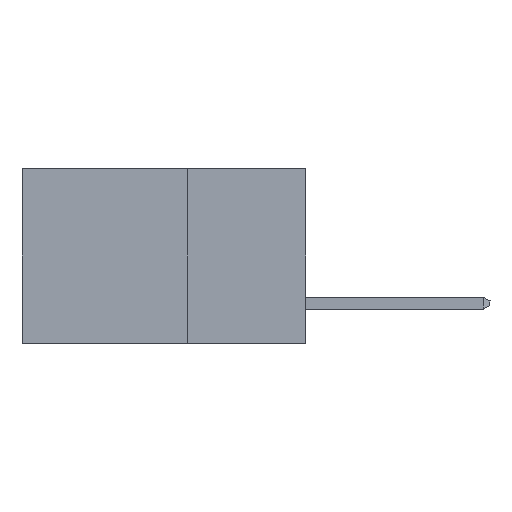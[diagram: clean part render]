
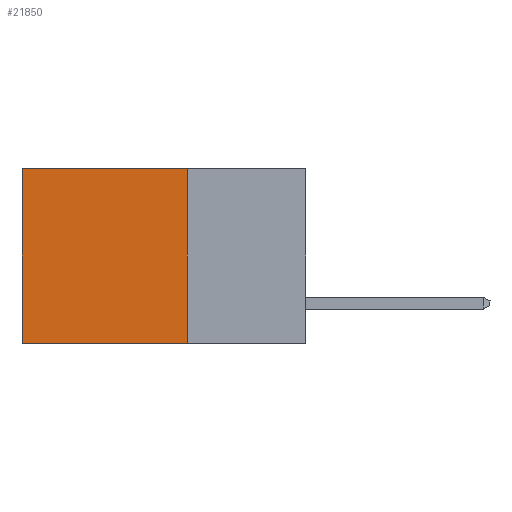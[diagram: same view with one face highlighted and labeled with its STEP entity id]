
A CAD part, left-side view. The second image highlights one B-rep face of the part: STEP entity #21850.
In plain terms, the highlighted planar face has unit normal (-1, 0, 0).
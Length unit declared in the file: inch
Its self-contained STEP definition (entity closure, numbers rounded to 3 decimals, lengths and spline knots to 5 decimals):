
#403 = VERTEX_POINT ( 'NONE', #14702 ) ;
#495 = AXIS2_PLACEMENT_3D ( 'NONE', #4971, #12656, #16238 ) ;
#599 = FACE_OUTER_BOUND ( 'NONE', #5117, .T. ) ;
#920 = DIRECTION ( 'NONE',  ( 0., 1., 0. ) ) ;
#1030 = EDGE_CURVE ( 'NONE', #403, #8289, #4589, .T. ) ;
#1401 = ORIENTED_EDGE ( 'NONE', *, *, #21392, .T. ) ;
#2047 = VECTOR ( 'NONE', #920, 39.37008 ) ;
#2135 = VECTOR ( 'NONE', #2304, 39.37008 ) ;
#2195 = LINE ( 'NONE', #9059, #6156 ) ;
#2304 = DIRECTION ( 'NONE',  ( 0., 0., -1. ) ) ;
#2977 = VERTEX_POINT ( 'NONE', #5341 ) ;
#3585 = ORIENTED_EDGE ( 'NONE', *, *, #11173, .F. ) ;
#4224 = EDGE_CURVE ( 'NONE', #2977, #8289, #2195, .T. ) ;
#4589 = LINE ( 'NONE', #7363, #6843 ) ;
#4674 = ORIENTED_EDGE ( 'NONE', *, *, #4224, .T. ) ;
#4971 = CARTESIAN_POINT ( 'NONE',  ( 0.298, 0.25, 0. ) ) ;
#5117 = EDGE_LOOP ( 'NONE', ( #4674, #22219, #3585, #1401 ) ) ;
#5341 = CARTESIAN_POINT ( 'NONE',  ( 0.298, 0.6, 0. ) ) ;
#6156 = VECTOR ( 'NONE', #7333, 39.37008 ) ;
#6843 = VECTOR ( 'NONE', #21718, 39.37008 ) ;
#7333 = DIRECTION ( 'NONE',  ( 0., 0., -1. ) ) ;
#7363 = CARTESIAN_POINT ( 'NONE',  ( 0.298, 0.25, -0.37 ) ) ;
#8289 = VERTEX_POINT ( 'NONE', #12252 ) ;
#8605 = LINE ( 'NONE', #20044, #2135 ) ;
#9059 = CARTESIAN_POINT ( 'NONE',  ( 0.298, 0.6, 0. ) ) ;
#10202 = LINE ( 'NONE', #13437, #2047 ) ;
#11173 = EDGE_CURVE ( 'NONE', #15555, #403, #8605, .T. ) ;
#12252 = CARTESIAN_POINT ( 'NONE',  ( 0.298, 0.6, -0.37 ) ) ;
#12656 = DIRECTION ( 'NONE',  ( 1., 0., 0. ) ) ;
#13437 = CARTESIAN_POINT ( 'NONE',  ( 0.298, 0.25, 0. ) ) ;
#14702 = CARTESIAN_POINT ( 'NONE',  ( 0.298, 0.25, -0.37 ) ) ;
#15555 = VERTEX_POINT ( 'NONE', #23233 ) ;
#16238 = DIRECTION ( 'NONE',  ( 0., 0., -1. ) ) ;
#17942 = PLANE ( 'NONE',  #495 ) ;
#20044 = CARTESIAN_POINT ( 'NONE',  ( 0.298, 0.25, 0. ) ) ;
#21392 = EDGE_CURVE ( 'NONE', #15555, #2977, #10202, .T. ) ;
#21718 = DIRECTION ( 'NONE',  ( 0., 1., 0. ) ) ;
#21850 = ADVANCED_FACE ( 'NONE', ( #599 ), #17942, .F. ) ;
#22219 = ORIENTED_EDGE ( 'NONE', *, *, #1030, .F. ) ;
#23233 = CARTESIAN_POINT ( 'NONE',  ( 0.298, 0.25, 0. ) ) ;
